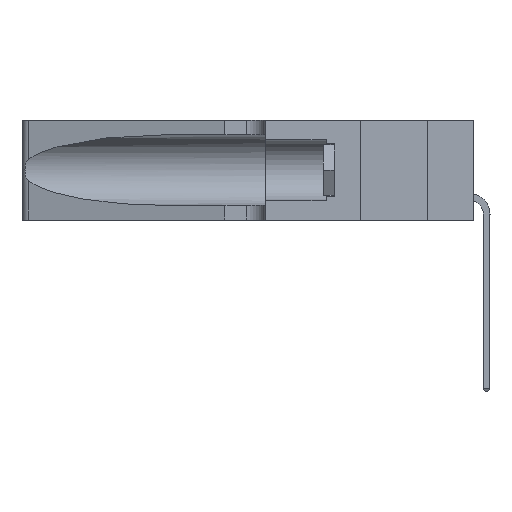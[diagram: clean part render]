
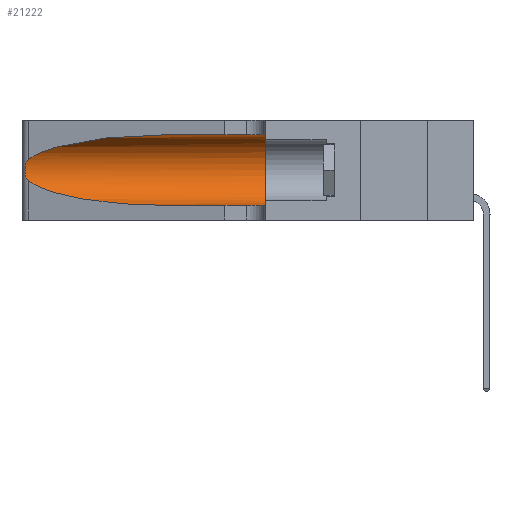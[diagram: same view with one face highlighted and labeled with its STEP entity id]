
A CAD part, left-side view. The second image highlights one B-rep face of the part: STEP entity #21222.
In plain terms, the highlighted cylindrical face has radius 3.308 mm (diameter 6.617 mm), a partial arc.
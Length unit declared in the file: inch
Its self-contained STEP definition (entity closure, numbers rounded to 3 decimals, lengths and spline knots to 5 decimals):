
#226 = EDGE_CURVE ( 'NONE', #47991, #18197, #39897, .T. ) ;
#849 = CIRCLE ( 'NONE', #16800, 0.13025 ) ;
#914 = ORIENTED_EDGE ( 'NONE', *, *, #8296, .T. ) ;
#1008 = ORIENTED_EDGE ( 'NONE', *, *, #9307, .T. ) ;
#1347 = EDGE_LOOP ( 'NONE', ( #16512, #14646, #914, #1008, #17403, #17481 ) ) ;
#1859 = CARTESIAN_POINT ( 'NONE',  ( 0.25487, 1.22718, 0.14631 ) ) ;
#2594 = CARTESIAN_POINT ( 'NONE',  ( 0.25639, 1.23186, 0.15144 ) ) ;
#2683 = CARTESIAN_POINT ( 'NONE',  ( 0.1305, 1.61858, 0.05475 ) ) ;
#4042 = CARTESIAN_POINT ( 'NONE',  ( 0.1305, 0.35, 0.05475 ) ) ;
#5660 = DIRECTION ( 'NONE',  ( 0., 1., 0. ) ) ;
#7206 = VERTEX_POINT ( 'NONE', #1859 ) ;
#8215 = CARTESIAN_POINT ( 'NONE',  ( 0.18966, 0.96281, 0.05475 ) ) ;
#8296 = EDGE_CURVE ( 'NONE', #7206, #25397, #9748, .T. ) ;
#9046 = CARTESIAN_POINT ( 'NONE',  ( 0.25487, 1.22718, 0.22369 ) ) ;
#9063 = LINE ( 'NONE', #17434, #13739 ) ;
#9131 = CARTESIAN_POINT ( 'NONE',  ( 0.1305, 0.72297, 0.31525 ) ) ;
#9307 = EDGE_CURVE ( 'NONE', #25397, #29269, #46344, .T. ) ;
#9748 =( BOUNDED_CURVE ( )  B_SPLINE_CURVE ( 3, ( #27412, #16835, #8215, #19296 ),
 .UNSPECIFIED., .F., .F. ) 
 B_SPLINE_CURVE_WITH_KNOTS ( ( 4, 4 ),
 ( 3.44316, 4.71239 ),
 .UNSPECIFIED. ) 
 CURVE ( )  GEOMETRIC_REPRESENTATION_ITEM ( )  RATIONAL_B_SPLINE_CURVE ( ( 1., 0.87, 0.87, 1. ) ) 
 REPRESENTATION_ITEM ( '' )  );
#10237 = CARTESIAN_POINT ( 'NONE',  ( 0.25789, 1.23486, 0.15765 ) ) ;
#10383 = CARTESIAN_POINT ( 'NONE',  ( 0.25487, 1.22718, 0.22369 ) ) ;
#13370 = VERTEX_POINT ( 'NONE', #36643 ) ;
#13739 = VECTOR ( 'NONE', #47209, 39.37008 ) ;
#14646 = ORIENTED_EDGE ( 'NONE', *, *, #32824, .T. ) ;
#14914 = VECTOR ( 'NONE', #38902, 39.37008 ) ;
#15842 = EDGE_CURVE ( 'NONE', #47991, #13370, #9063, .T. ) ;
#16512 = ORIENTED_EDGE ( 'NONE', *, *, #226, .T. ) ;
#16800 = AXIS2_PLACEMENT_3D ( 'NONE', #46491, #5660, #38852 ) ;
#16835 = CARTESIAN_POINT ( 'NONE',  ( 0.2373, 1.15595, 0.08982 ) ) ;
#17403 = ORIENTED_EDGE ( 'NONE', *, *, #31590, .F. ) ;
#17432 = FACE_OUTER_BOUND ( 'NONE', #1347, .T. ) ;
#17434 = CARTESIAN_POINT ( 'NONE',  ( 0.1305, 1.61858, 0.31525 ) ) ;
#17481 = ORIENTED_EDGE ( 'NONE', *, *, #15842, .F. ) ;
#18197 = VERTEX_POINT ( 'NONE', #46720 ) ;
#18840 = CARTESIAN_POINT ( 'NONE',  ( 0.1305, 1.61858, 0.185 ) ) ;
#19296 = CARTESIAN_POINT ( 'NONE',  ( 0.1305, 0.72297, 0.05475 ) ) ;
#20285 = CARTESIAN_POINT ( 'NONE',  ( 0.25555, 1.22993, 0.14849 ) ) ;
#21222 = ADVANCED_FACE ( 'NONE', ( #17432 ), #37799, .F. ) ;
#21444 = CARTESIAN_POINT ( 'NONE',  ( 0.25487, 1.22718, 0.14631 ) ) ;
#21601 = CARTESIAN_POINT ( 'NONE',  ( 0.25787, 1.23484, 0.2124 ) ) ;
#24857 = CARTESIAN_POINT ( 'NONE',  ( 0.26075, 1.23896, 0.19203 ) ) ;
#25397 = VERTEX_POINT ( 'NONE', #46976 ) ;
#26267 = AXIS2_PLACEMENT_3D ( 'NONE', #18840, #45005, #30544 ) ;
#27412 = CARTESIAN_POINT ( 'NONE',  ( 0.25487, 1.22718, 0.14631 ) ) ;
#29269 = VERTEX_POINT ( 'NONE', #4042 ) ;
#30544 = DIRECTION ( 'NONE',  ( 0., 0., -1. ) ) ;
#31296 = CARTESIAN_POINT ( 'NONE',  ( 0.18966, 0.96281, 0.31525 ) ) ;
#31590 = EDGE_CURVE ( 'NONE', #13370, #29269, #849, .T. ) ;
#32340 = CARTESIAN_POINT ( 'NONE',  ( 0.25639, 1.23184, 0.21858 ) ) ;
#32824 = EDGE_CURVE ( 'NONE', #18197, #7206, #41307, .T. ) ;
#35059 = CARTESIAN_POINT ( 'NONE',  ( 0.26075, 1.23896, 0.178 ) ) ;
#36059 = CARTESIAN_POINT ( 'NONE',  ( 0.26017, 1.23833, 0.17102 ) ) ;
#36643 = CARTESIAN_POINT ( 'NONE',  ( 0.1305, 0.35, 0.31525 ) ) ;
#37799 = CYLINDRICAL_SURFACE ( 'NONE', #26267, 0.13025 ) ;
#38852 = DIRECTION ( 'NONE',  ( 0., 0., 1. ) ) ;
#38902 = DIRECTION ( 'NONE',  ( 0., -1., 0. ) ) ;
#38985 = CARTESIAN_POINT ( 'NONE',  ( 0.2373, 1.15595, 0.28018 ) ) ;
#39897 =( BOUNDED_CURVE ( )  B_SPLINE_CURVE ( 3, ( #46115, #31296, #38985, #9046 ),
 .UNSPECIFIED., .F., .F. ) 
 B_SPLINE_CURVE_WITH_KNOTS ( ( 4, 4 ),
 ( 1.5708, 2.84003 ),
 .UNSPECIFIED. ) 
 CURVE ( )  GEOMETRIC_REPRESENTATION_ITEM ( )  RATIONAL_B_SPLINE_CURVE ( ( 1., 0.87, 0.87, 1. ) ) 
 REPRESENTATION_ITEM ( '' )  );
#39995 = CARTESIAN_POINT ( 'NONE',  ( 0.26018, 1.23835, 0.19895 ) ) ;
#41307 = B_SPLINE_CURVE_WITH_KNOTS ( 'NONE', 3,
 ( #10383, #43887, #32340, #21601, #42705, #39995, #24857, #35059, #36059, #43723, #10237, #2594, #20285, #21444 ),
 .UNSPECIFIED., .F., .F.,
 ( 4, 2, 2, 2, 2, 2, 4 ),
 ( 0., 0.00027, 0.00053, 0.00107, 0.0016, 0.00187, 0.00214 ),
 .UNSPECIFIED. ) ;
#42705 = CARTESIAN_POINT ( 'NONE',  ( 0.25854, 1.2359, 0.20912 ) ) ;
#43723 = CARTESIAN_POINT ( 'NONE',  ( 0.25856, 1.23593, 0.16098 ) ) ;
#43887 = CARTESIAN_POINT ( 'NONE',  ( 0.25555, 1.22994, 0.2215 ) ) ;
#45005 = DIRECTION ( 'NONE',  ( 0., -1., 0. ) ) ;
#46115 = CARTESIAN_POINT ( 'NONE',  ( 0.1305, 0.72297, 0.31525 ) ) ;
#46344 = LINE ( 'NONE', #2683, #14914 ) ;
#46491 = CARTESIAN_POINT ( 'NONE',  ( 0.1305, 0.35, 0.185 ) ) ;
#46720 = CARTESIAN_POINT ( 'NONE',  ( 0.25487, 1.22718, 0.22369 ) ) ;
#46976 = CARTESIAN_POINT ( 'NONE',  ( 0.1305, 0.72297, 0.05475 ) ) ;
#47209 = DIRECTION ( 'NONE',  ( 0., -1., 0. ) ) ;
#47991 = VERTEX_POINT ( 'NONE', #9131 ) ;
